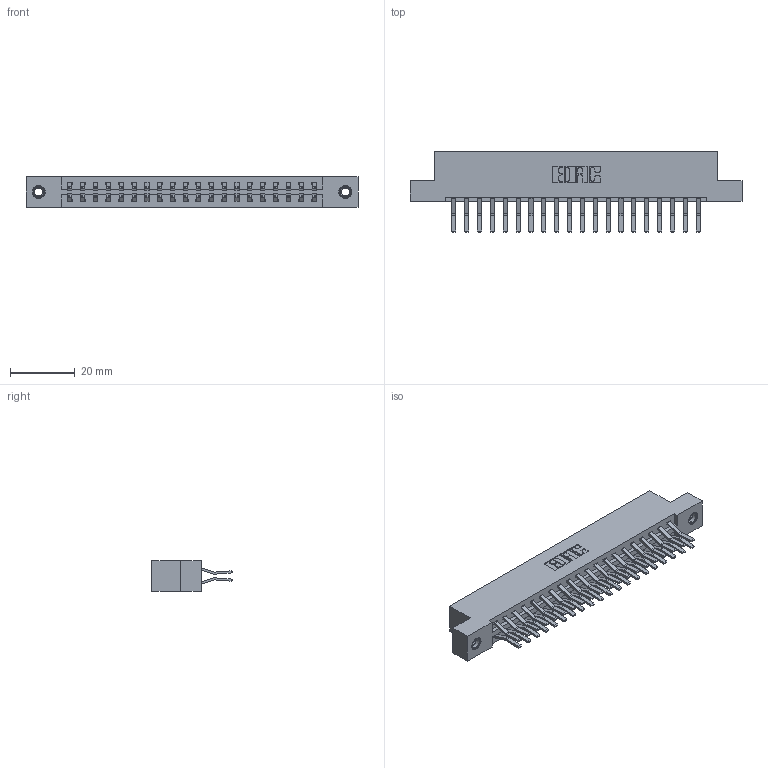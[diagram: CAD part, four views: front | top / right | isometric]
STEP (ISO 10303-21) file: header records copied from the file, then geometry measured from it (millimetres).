
FILE_DESCRIPTION (( 'STEP AP203' ), '1' );
FILE_NAME ('387-040-560-207.STEP', '2018-09-19T17:32:31', ( '' ), ( '' ), 'SwSTEP 2.0', 'SolidWorks 2016', '' );
FILE_SCHEMA (( 'CONFIG_CONTROL_DESIGN' ));
Length unit declared in the file: inch
Products named in the file (4): 337 Part_Flush Mounting Lugs - 0.156 Dia-TI; 345-292-001_560 Tail; 345-250-001_345-250-005-103; 387-040-560-207
Assembly tree (43 placements, depth 2):
  387-040-560-207
    337 Part_Flush Mounting Lugs - 0.156 Dia-TI
    345-292-001_560 Tail  x40
    345-250-001_345-250-005-103  x2
Bounding box: 102.26 x 24.78 x 9.4 mm (x, y, z)
Volume: 10732.8 mm3; surface area: 12714.6 mm2
Topology: 43 solids, 43 shells, 2414 faces, 7127 edges, 4690 vertices
Faces by surface type: plane 1622, cylinder 776, cone 12, torus 4
Entity records: 19626 total; most frequent: CARTESIAN_POINT 3305, ORIENTED_EDGE 3234, DIRECTION 2887, EDGE_CURVE 1617, VECTOR 1465, LINE 1465, VERTEX_POINT 1072, AXIS2_PLACEMENT_3D 711
